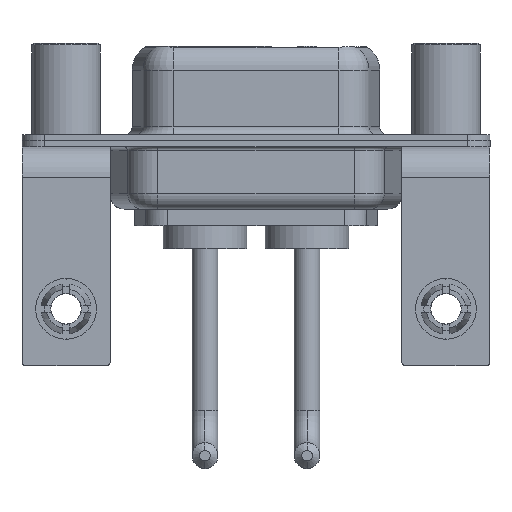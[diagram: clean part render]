
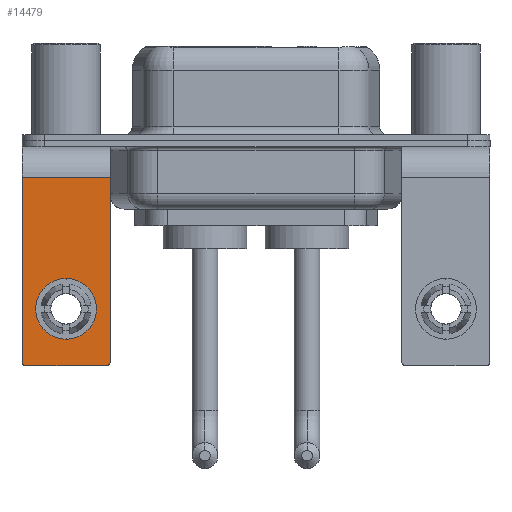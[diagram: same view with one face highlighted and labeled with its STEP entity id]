
A CAD part, front view. The second image highlights one B-rep face of the part: STEP entity #14479.
In plain terms, the highlighted planar face has unit normal (0, -1, 0).
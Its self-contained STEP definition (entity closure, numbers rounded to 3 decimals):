
#206 = CARTESIAN_POINT ( 'NONE',  ( 0., -6.25, -11.07 ) ) ;
#373 = ORIENTED_EDGE ( 'NONE', *, *, #14919, .T. ) ;
#808 = DIRECTION ( 'NONE',  ( 0., -1., 0. ) ) ;
#858 = EDGE_CURVE ( 'NONE', #3701, #13320, #10176, .T. ) ;
#955 = EDGE_LOOP ( 'NONE', ( #14655, #1079 ) ) ;
#1079 = ORIENTED_EDGE ( 'NONE', *, *, #5209, .T. ) ;
#1091 = FACE_BOUND ( 'NONE', #955, .T. ) ;
#1625 = VERTEX_POINT ( 'NONE', #9716 ) ;
#1693 = CARTESIAN_POINT ( 'NONE',  ( 2.9, -6.25, -2.4 ) ) ;
#2029 = CARTESIAN_POINT ( 'NONE',  ( 2.65, -6.25, -14.8 ) ) ;
#2062 = VECTOR ( 'NONE', #3913, 1000. ) ;
#2577 = DIRECTION ( 'NONE',  ( 0., 0., 1. ) ) ;
#3157 = DIRECTION ( 'NONE',  ( -1., 0., 0. ) ) ;
#3460 = CARTESIAN_POINT ( 'NONE',  ( -2.9, -6.25, -2.4 ) ) ;
#3701 = VERTEX_POINT ( 'NONE', #11188 ) ;
#3743 = AXIS2_PLACEMENT_3D ( 'NONE', #10520, #808, #10613 ) ;
#3913 = DIRECTION ( 'NONE',  ( -1., 0., 0. ) ) ;
#4448 = LINE ( 'NONE', #1693, #13071 ) ;
#4788 = CARTESIAN_POINT ( 'NONE',  ( -2.65, -6.25, -14.55 ) ) ;
#5209 = EDGE_CURVE ( 'NONE', #13320, #3701, #7180, .T. ) ;
#5507 = DIRECTION ( 'NONE',  ( 0., 0., 1. ) ) ;
#5593 = DIRECTION ( 'NONE',  ( 0., 1., 0. ) ) ;
#5846 = DIRECTION ( 'NONE',  ( 0., 0., 1. ) ) ;
#5964 = DIRECTION ( 'NONE',  ( 0., 1., 0. ) ) ;
#5989 = ORIENTED_EDGE ( 'NONE', *, *, #17380, .F. ) ;
#6103 = VERTEX_POINT ( 'NONE', #14988 ) ;
#6208 = CARTESIAN_POINT ( 'NONE',  ( 2.9, -6.25, -14.55 ) ) ;
#6218 = DIRECTION ( 'NONE',  ( 0., 0., 1. ) ) ;
#6465 = FACE_OUTER_BOUND ( 'NONE', #8246, .T. ) ;
#7180 = CIRCLE ( 'NONE', #9151, 2. ) ;
#7367 = CARTESIAN_POINT ( 'NONE',  ( 0., -6.25, -11.07 ) ) ;
#7397 = CARTESIAN_POINT ( 'NONE',  ( -2.65, -6.25, -14.8 ) ) ;
#7472 = LINE ( 'NONE', #14177, #13774 ) ;
#8246 = EDGE_LOOP ( 'NONE', ( #9384, #11041, #13455, #373, #5989, #13374 ) ) ;
#8530 = VERTEX_POINT ( 'NONE', #14434 ) ;
#8776 = LINE ( 'NONE', #16796, #2062 ) ;
#9151 = AXIS2_PLACEMENT_3D ( 'NONE', #7367, #5964, #6218 ) ;
#9384 = ORIENTED_EDGE ( 'NONE', *, *, #14827, .T. ) ;
#9440 = CIRCLE ( 'NONE', #12541, 0.25 ) ;
#9716 = CARTESIAN_POINT ( 'NONE',  ( 2.9, -6.25, -2.4 ) ) ;
#10173 = DIRECTION ( 'NONE',  ( 0., 0., -1. ) ) ;
#10176 = CIRCLE ( 'NONE', #16939, 2. ) ;
#10520 = CARTESIAN_POINT ( 'NONE',  ( 2.65, -6.25, -14.55 ) ) ;
#10540 = CARTESIAN_POINT ( 'NONE',  ( 2.9, -6.25, -2.4 ) ) ;
#10613 = DIRECTION ( 'NONE',  ( 0., 0., 1. ) ) ;
#11041 = ORIENTED_EDGE ( 'NONE', *, *, #16316, .T. ) ;
#11188 = CARTESIAN_POINT ( 'NONE',  ( 0., -6.25, -13.07 ) ) ;
#11475 = CARTESIAN_POINT ( 'NONE',  ( 0., -6.25, -9.07 ) ) ;
#11629 = AXIS2_PLACEMENT_3D ( 'NONE', #10540, #15920, #2577 ) ;
#11648 = VECTOR ( 'NONE', #10173, 1000. ) ;
#11886 = VERTEX_POINT ( 'NONE', #7397 ) ;
#12541 = AXIS2_PLACEMENT_3D ( 'NONE', #4788, #16523, #5846 ) ;
#13071 = VECTOR ( 'NONE', #15116, 1000. ) ;
#13320 = VERTEX_POINT ( 'NONE', #11475 ) ;
#13374 = ORIENTED_EDGE ( 'NONE', *, *, #13714, .T. ) ;
#13455 = ORIENTED_EDGE ( 'NONE', *, *, #15869, .F. ) ;
#13714 = EDGE_CURVE ( 'NONE', #1625, #6103, #7472, .T. ) ;
#13774 = VECTOR ( 'NONE', #3157, 1000. ) ;
#14167 = CIRCLE ( 'NONE', #3743, 0.25 ) ;
#14177 = CARTESIAN_POINT ( 'NONE',  ( 2.9, -6.25, -2.4 ) ) ;
#14434 = CARTESIAN_POINT ( 'NONE',  ( -2.9, -6.25, -14.55 ) ) ;
#14479 = ADVANCED_FACE ( 'NONE', ( #1091, #6465 ), #17237, .F. ) ;
#14655 = ORIENTED_EDGE ( 'NONE', *, *, #858, .T. ) ;
#14695 = VERTEX_POINT ( 'NONE', #2029 ) ;
#14827 = EDGE_CURVE ( 'NONE', #6103, #8530, #15901, .T. ) ;
#14919 = EDGE_CURVE ( 'NONE', #14695, #17141, #14167, .T. ) ;
#14988 = CARTESIAN_POINT ( 'NONE',  ( -2.9, -6.25, -2.4 ) ) ;
#15116 = DIRECTION ( 'NONE',  ( 0., 0., -1. ) ) ;
#15869 = EDGE_CURVE ( 'NONE', #14695, #11886, #8776, .T. ) ;
#15901 = LINE ( 'NONE', #3460, #11648 ) ;
#15920 = DIRECTION ( 'NONE',  ( 0., 1., 0. ) ) ;
#16316 = EDGE_CURVE ( 'NONE', #8530, #11886, #9440, .T. ) ;
#16523 = DIRECTION ( 'NONE',  ( 0., -1., 0. ) ) ;
#16796 = CARTESIAN_POINT ( 'NONE',  ( 2.9, -6.25, -14.8 ) ) ;
#16939 = AXIS2_PLACEMENT_3D ( 'NONE', #206, #5593, #5507 ) ;
#17141 = VERTEX_POINT ( 'NONE', #6208 ) ;
#17237 = PLANE ( 'NONE',  #11629 ) ;
#17380 = EDGE_CURVE ( 'NONE', #1625, #17141, #4448, .T. ) ;
